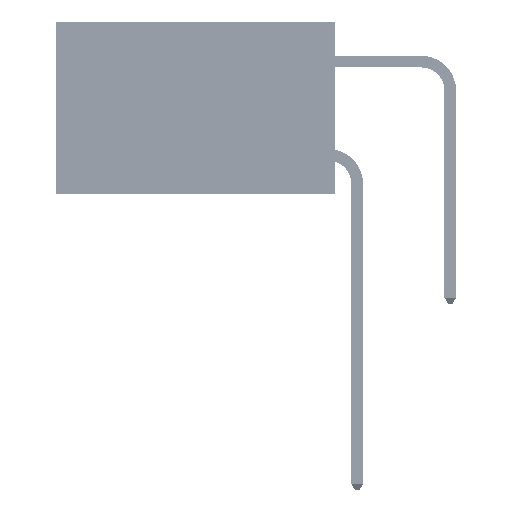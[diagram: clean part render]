
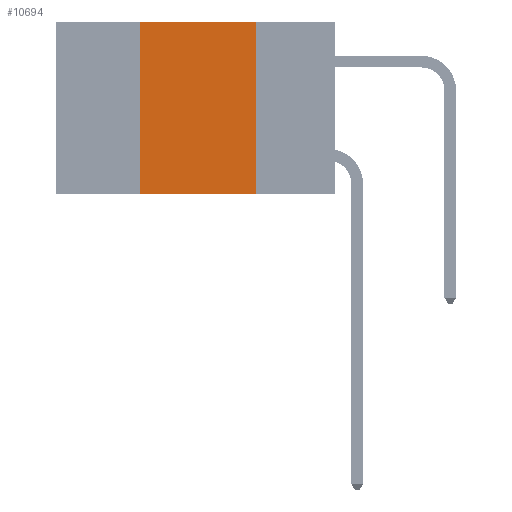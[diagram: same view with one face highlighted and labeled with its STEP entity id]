
A CAD part, left-side view. The second image highlights one B-rep face of the part: STEP entity #10694.
In plain terms, the highlighted planar face has unit normal (-1, 0, 0).
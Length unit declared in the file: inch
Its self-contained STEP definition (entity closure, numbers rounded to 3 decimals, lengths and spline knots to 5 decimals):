
#40 = DIRECTION ( 'NONE',  ( 0., -1., 0. ) ) ;
#1865 = LINE ( 'NONE', #2101, #32761 ) ;
#2101 = CARTESIAN_POINT ( 'NONE',  ( 0., 0.42, 0. ) ) ;
#4459 = DIRECTION ( 'NONE',  ( 0., 0., -1. ) ) ;
#6149 = DIRECTION ( 'NONE',  ( 0., 0., 1. ) ) ;
#8820 = LINE ( 'NONE', #48304, #39721 ) ;
#9266 = VERTEX_POINT ( 'NONE', #21508 ) ;
#10694 = ADVANCED_FACE ( 'NONE', ( #34947 ), #12423, .F. ) ;
#12423 = PLANE ( 'NONE',  #24283 ) ;
#12837 = CARTESIAN_POINT ( 'NONE',  ( 0., 0.42, -0.37 ) ) ;
#13310 = EDGE_CURVE ( 'NONE', #22666, #23935, #36613, .T. ) ;
#13442 = EDGE_CURVE ( 'NONE', #9266, #22666, #8820, .T. ) ;
#14657 = EDGE_CURVE ( 'NONE', #42909, #23935, #38416, .T. ) ;
#14935 = CARTESIAN_POINT ( 'NONE',  ( 0., 0.6, -0.37 ) ) ;
#15105 = DIRECTION ( 'NONE',  ( 0., -1., 0. ) ) ;
#15725 = VECTOR ( 'NONE', #15105, 39.37008 ) ;
#15900 = CARTESIAN_POINT ( 'NONE',  ( 0., 0.17, -0.37 ) ) ;
#17722 = ORIENTED_EDGE ( 'NONE', *, *, #13442, .F. ) ;
#21508 = CARTESIAN_POINT ( 'NONE',  ( 0., 0.42, 0. ) ) ;
#21673 = CARTESIAN_POINT ( 'NONE',  ( 0., 0.17, 0. ) ) ;
#22666 = VERTEX_POINT ( 'NONE', #43999 ) ;
#23935 = VERTEX_POINT ( 'NONE', #15900 ) ;
#24283 = AXIS2_PLACEMENT_3D ( 'NONE', #40582, #28592, #4459 ) ;
#25707 = DIRECTION ( 'NONE',  ( 0., 0., -1. ) ) ;
#28592 = DIRECTION ( 'NONE',  ( 1., 0., 0. ) ) ;
#30149 = ORIENTED_EDGE ( 'NONE', *, *, #14657, .T. ) ;
#32761 = VECTOR ( 'NONE', #6149, 39.37008 ) ;
#33467 = ORIENTED_EDGE ( 'NONE', *, *, #13310, .F. ) ;
#34947 = FACE_OUTER_BOUND ( 'NONE', #51148, .T. ) ;
#35339 = VECTOR ( 'NONE', #25707, 39.37008 ) ;
#35407 = EDGE_CURVE ( 'NONE', #42909, #9266, #1865, .T. ) ;
#36613 = LINE ( 'NONE', #21673, #35339 ) ;
#36860 = ORIENTED_EDGE ( 'NONE', *, *, #35407, .F. ) ;
#38416 = LINE ( 'NONE', #14935, #15725 ) ;
#39721 = VECTOR ( 'NONE', #40, 39.37008 ) ;
#40582 = CARTESIAN_POINT ( 'NONE',  ( 0., 0.6, 0. ) ) ;
#42909 = VERTEX_POINT ( 'NONE', #12837 ) ;
#43999 = CARTESIAN_POINT ( 'NONE',  ( 0., 0.17, 0. ) ) ;
#48304 = CARTESIAN_POINT ( 'NONE',  ( 0., 0.6, 0. ) ) ;
#51148 = EDGE_LOOP ( 'NONE', ( #33467, #17722, #36860, #30149 ) ) ;
